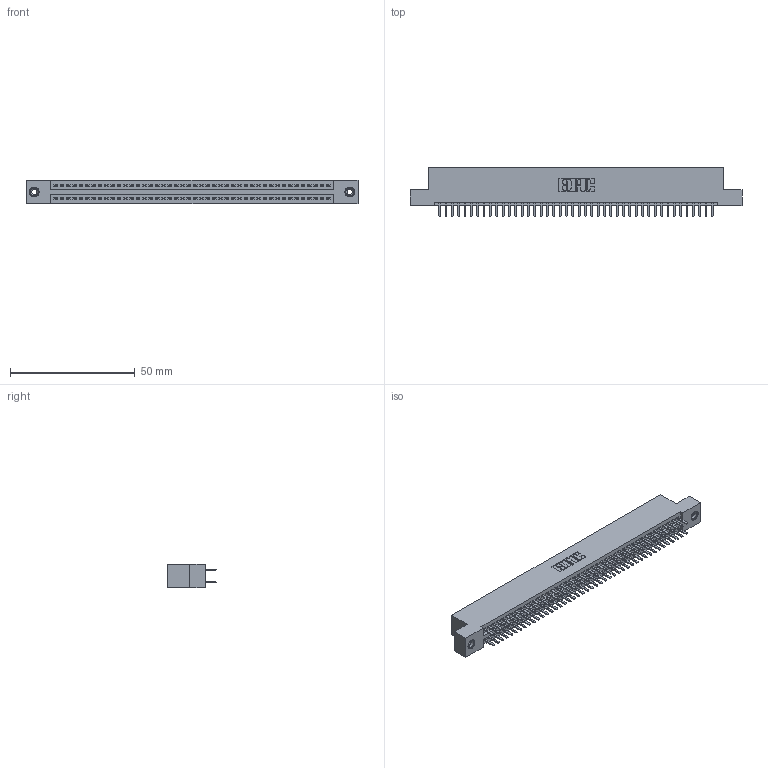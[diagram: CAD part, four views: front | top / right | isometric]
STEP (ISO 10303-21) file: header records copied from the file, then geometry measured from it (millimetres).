
FILE_DESCRIPTION (( 'STEP AP203' ), '1' );
FILE_NAME ('395-088-520-208.STEP', '2019-10-25T13:09:33', ( '' ), ( '' ), 'SwSTEP 2.0', 'SolidWorks 2016', '' );
FILE_SCHEMA (( 'CONFIG_CONTROL_DESIGN' ));
Length unit declared in the file: inch
Products named in the file (4): 345-292-001_345-293-120; 345-250-001_345-250-003-102; 395-088-520-208; 345 Part_Flush Mounting Lugs - 0.156 Dia-TI
Assembly tree (91 placements, depth 2):
  395-088-520-208
    345 Part_Flush Mounting Lugs - 0.156 Dia-TI
    345-292-001_345-293-120  x88
    345-250-001_345-250-003-102  x2
Bounding box: 132.97 x 19.68 x 9.4 mm (x, y, z)
Volume: 12890.1 mm3; surface area: 19023.6 mm2
Topology: 91 solids, 91 shells, 4938 faces, 14293 edges, 9286 vertices
Faces by surface type: plane 3192, cylinder 1730, cone 12, torus 4
Entity records: 35554 total; most frequent: CARTESIAN_POINT 5951, ORIENTED_EDGE 5866, DIRECTION 5259, EDGE_CURVE 2933, LINE 2601, VECTOR 2601, VERTEX_POINT 1948, AXIS2_PLACEMENT_3D 1329
